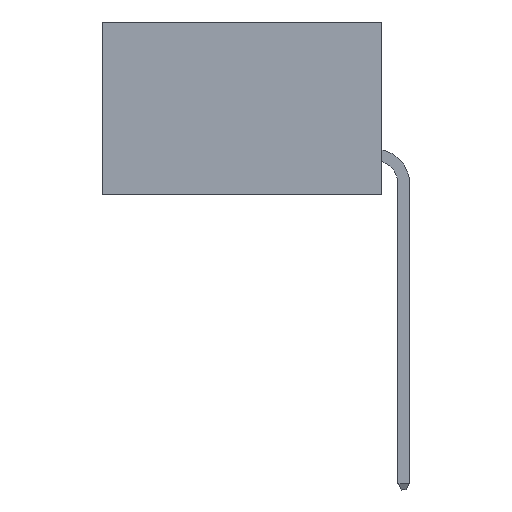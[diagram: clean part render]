
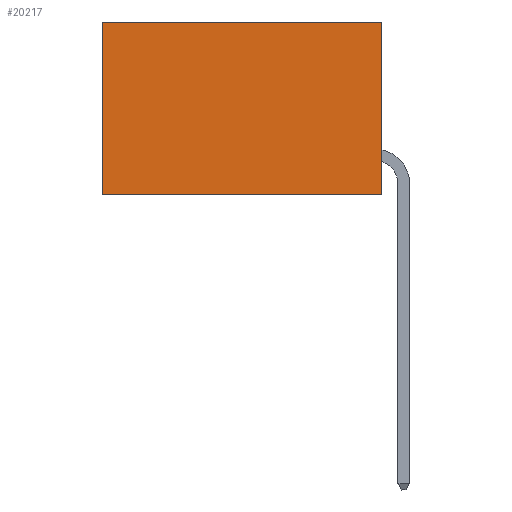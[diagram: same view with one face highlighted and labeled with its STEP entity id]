
A CAD part, left-side view. The second image highlights one B-rep face of the part: STEP entity #20217.
In plain terms, the highlighted planar face has unit normal (-1, 0, 0).
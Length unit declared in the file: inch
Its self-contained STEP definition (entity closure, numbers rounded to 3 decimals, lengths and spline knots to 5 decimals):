
#552 = CARTESIAN_POINT ( 'NONE',  ( 0.2875, 0.6, 0. ) ) ;
#988 = DIRECTION ( 'NONE',  ( 0., 0., -1. ) ) ;
#1046 = ORIENTED_EDGE ( 'NONE', *, *, #20674, .T. ) ;
#1571 = LINE ( 'NONE', #31678, #21750 ) ;
#4772 = CARTESIAN_POINT ( 'NONE',  ( 0.2875, 0., 0. ) ) ;
#6902 = CARTESIAN_POINT ( 'NONE',  ( 0.2875, 0., 0. ) ) ;
#7878 = VECTOR ( 'NONE', #24619, 39.37008 ) ;
#9471 = DIRECTION ( 'NONE',  ( 1., 0., 0. ) ) ;
#10296 = VERTEX_POINT ( 'NONE', #4772 ) ;
#10568 = EDGE_CURVE ( 'NONE', #17374, #10792, #30227, .T. ) ;
#10792 = VERTEX_POINT ( 'NONE', #32019 ) ;
#11066 = VECTOR ( 'NONE', #988, 39.37008 ) ;
#11449 = EDGE_CURVE ( 'NONE', #17015, #10792, #15332, .T. ) ;
#14452 = ORIENTED_EDGE ( 'NONE', *, *, #21491, .F. ) ;
#15332 = LINE ( 'NONE', #22111, #7878 ) ;
#15686 = EDGE_LOOP ( 'NONE', ( #22185, #18628, #14452, #1046 ) ) ;
#15964 = FACE_OUTER_BOUND ( 'NONE', #15686, .T. ) ;
#16215 = CARTESIAN_POINT ( 'NONE',  ( 0.2875, 0., 0. ) ) ;
#16915 = PLANE ( 'NONE',  #18165 ) ;
#17015 = VERTEX_POINT ( 'NONE', #19436 ) ;
#17374 = VERTEX_POINT ( 'NONE', #552 ) ;
#18165 = AXIS2_PLACEMENT_3D ( 'NONE', #6902, #9471, #26944 ) ;
#18628 = ORIENTED_EDGE ( 'NONE', *, *, #11449, .F. ) ;
#18732 = CARTESIAN_POINT ( 'NONE',  ( 0.2875, 0.6, 0. ) ) ;
#18745 = DIRECTION ( 'NONE',  ( 0., 1., 0. ) ) ;
#19436 = CARTESIAN_POINT ( 'NONE',  ( 0.2875, 0., -0.37 ) ) ;
#20217 = ADVANCED_FACE ( 'NONE', ( #15964 ), #16915, .F. ) ;
#20674 = EDGE_CURVE ( 'NONE', #10296, #17374, #21814, .T. ) ;
#21491 = EDGE_CURVE ( 'NONE', #10296, #17015, #1571, .T. ) ;
#21750 = VECTOR ( 'NONE', #29266, 39.37008 ) ;
#21814 = LINE ( 'NONE', #16215, #28422 ) ;
#22111 = CARTESIAN_POINT ( 'NONE',  ( 0.2875, 0., -0.37 ) ) ;
#22185 = ORIENTED_EDGE ( 'NONE', *, *, #10568, .T. ) ;
#24619 = DIRECTION ( 'NONE',  ( 0., 1., 0. ) ) ;
#26944 = DIRECTION ( 'NONE',  ( 0., 0., -1. ) ) ;
#28422 = VECTOR ( 'NONE', #18745, 39.37008 ) ;
#29266 = DIRECTION ( 'NONE',  ( 0., 0., -1. ) ) ;
#30227 = LINE ( 'NONE', #18732, #11066 ) ;
#31678 = CARTESIAN_POINT ( 'NONE',  ( 0.2875, 0., 0. ) ) ;
#32019 = CARTESIAN_POINT ( 'NONE',  ( 0.2875, 0.6, -0.37 ) ) ;
